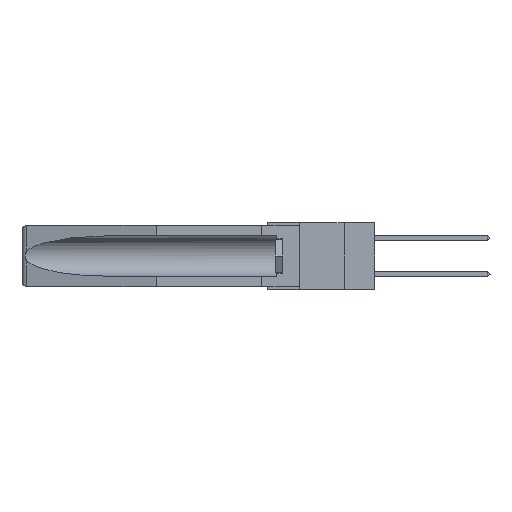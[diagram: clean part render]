
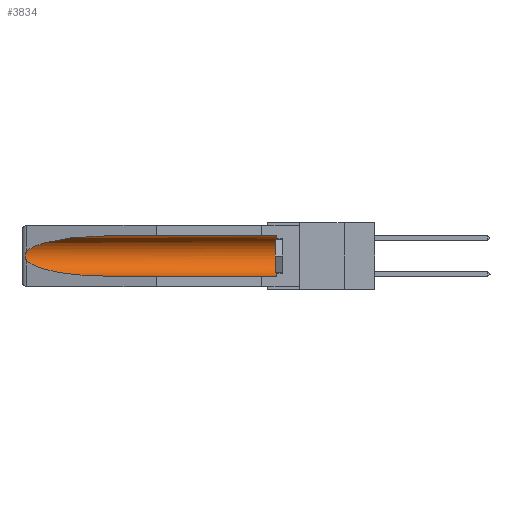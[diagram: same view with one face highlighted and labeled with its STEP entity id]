
A CAD part, left-side view. The second image highlights one B-rep face of the part: STEP entity #3834.
In plain terms, the highlighted cylindrical face has radius 2.857 mm (diameter 5.715 mm), a partial arc.
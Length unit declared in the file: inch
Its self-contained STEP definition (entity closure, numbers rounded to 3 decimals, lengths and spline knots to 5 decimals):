
#328 = ORIENTED_EDGE ( 'NONE', *, *, #12230, .T. ) ;
#489 = CARTESIAN_POINT ( 'NONE',  ( 0.155, 0.126, -0.284 ) ) ;
#1151 = AXIS2_PLACEMENT_3D ( 'NONE', #7534, #4968, #14448 ) ;
#1453 = EDGE_CURVE ( 'NONE', #27020, #3068, #8650, .T. ) ;
#1530 = CARTESIAN_POINT ( 'NONE',  ( 0.2673, 1.53269, -0.17917 ) ) ;
#1660 = CARTESIAN_POINT ( 'NONE',  ( 0.26537, 1.52718, -0.19328 ) ) ;
#2559 = CARTESIAN_POINT ( 'NONE',  ( 0.21114, 1.30732, -0.059 ) ) ;
#3068 = VERTEX_POINT ( 'NONE', #8744 ) ;
#3500 = VERTEX_POINT ( 'NONE', #16762 ) ;
#3834 = ADVANCED_FACE ( 'NONE', ( #11107 ), #24157, .F. ) ;
#3951 = CARTESIAN_POINT ( 'NONE',  ( 0.25451, 1.48313, -0.24835 ) ) ;
#4860 = CARTESIAN_POINT ( 'NONE',  ( 0.26537, 1.52718, -0.14972 ) ) ;
#4968 = DIRECTION ( 'NONE',  ( 0., -1., 0. ) ) ;
#6012 = CARTESIAN_POINT ( 'NONE',  ( 0.26537, 1.52718, -0.19328 ) ) ;
#6924 = ORIENTED_EDGE ( 'NONE', *, *, #9875, .T. ) ;
#7005 = ORIENTED_EDGE ( 'NONE', *, *, #20177, .T. ) ;
#7534 = CARTESIAN_POINT ( 'NONE',  ( 0.155, 0.126, -0.1715 ) ) ;
#8206 = CARTESIAN_POINT ( 'NONE',  ( 0.26537, 1.52718, -0.14972 ) ) ;
#8302 = CARTESIAN_POINT ( 'NONE',  ( 0.2675, 1.53308, -0.16763 ) ) ;
#8340 = CARTESIAN_POINT ( 'NONE',  ( 0.155, 1.07973, -0.284 ) ) ;
#8650 = CIRCLE ( 'NONE', #1151, 0.1125 ) ;
#8744 = CARTESIAN_POINT ( 'NONE',  ( 0.155, 0.126, -0.059 ) ) ;
#9875 = EDGE_CURVE ( 'NONE', #3500, #29275, #27918, .T. ) ;
#10318 = CARTESIAN_POINT ( 'NONE',  ( 0.21114, 1.30732, -0.284 ) ) ;
#10453 = LINE ( 'NONE', #14992, #12602 ) ;
#10569 = CARTESIAN_POINT ( 'NONE',  ( 0.2675, 1.53308, -0.17534 ) ) ;
#10689 = DIRECTION ( 'NONE',  ( 0., 1., 0. ) ) ;
#11107 = FACE_OUTER_BOUND ( 'NONE', #26128, .T. ) ;
#11844 = EDGE_CURVE ( 'NONE', #14674, #22599, #17428, .T. ) ;
#12136 = B_SPLINE_CURVE_WITH_KNOTS ( 'NONE', 3,
 ( #8206, #26309, #24010, #19602, #8302, #10569, #1530, #12877, #17172, #6012 ),
 .UNSPECIFIED., .F., .F.,
 ( 4, 2, 2, 2, 4 ),
 ( 0., 0.00029, 0.00058, 0.00087, 0.00117 ),
 .UNSPECIFIED. ) ;
#12230 = EDGE_CURVE ( 'NONE', #29275, #14674, #12136, .T. ) ;
#12359 = ORIENTED_EDGE ( 'NONE', *, *, #16674, .F. ) ;
#12436 = LINE ( 'NONE', #12764, #19887 ) ;
#12602 = VECTOR ( 'NONE', #10689, 39.37008 ) ;
#12764 = CARTESIAN_POINT ( 'NONE',  ( 0.155, -0.30754, -0.284 ) ) ;
#12877 = CARTESIAN_POINT ( 'NONE',  ( 0.26655, 1.53094, -0.18657 ) ) ;
#13582 = DIRECTION ( 'NONE',  ( 0., 1., 0. ) ) ;
#14448 = DIRECTION ( 'NONE',  ( 0., 0., 1. ) ) ;
#14674 = VERTEX_POINT ( 'NONE', #24189 ) ;
#14992 = CARTESIAN_POINT ( 'NONE',  ( 0.155, -0.30754, -0.059 ) ) ;
#15958 = CARTESIAN_POINT ( 'NONE',  ( 0.155, -0.30754, -0.1715 ) ) ;
#16184 = CARTESIAN_POINT ( 'NONE',  ( 0.155, 1.07973, -0.059 ) ) ;
#16664 = ORIENTED_EDGE ( 'NONE', *, *, #1453, .T. ) ;
#16674 = EDGE_CURVE ( 'NONE', #27020, #22599, #12436, .T. ) ;
#16762 = CARTESIAN_POINT ( 'NONE',  ( 0.155, 1.07973, -0.059 ) ) ;
#17172 = CARTESIAN_POINT ( 'NONE',  ( 0.26597, 1.5296, -0.19026 ) ) ;
#17428 =( BOUNDED_CURVE ( )  B_SPLINE_CURVE ( 3, ( #1660, #3951, #10318, #8340 ),
 .UNSPECIFIED., .F., .F. ) 
 B_SPLINE_CURVE_WITH_KNOTS ( ( 4, 4 ),
 ( 0.1948, 1.5708 ),
 .UNSPECIFIED. ) 
 CURVE ( )  GEOMETRIC_REPRESENTATION_ITEM ( )  RATIONAL_B_SPLINE_CURVE ( ( 1., 0.848, 0.848, 1. ) ) 
 REPRESENTATION_ITEM ( '' )  );
#18464 = CARTESIAN_POINT ( 'NONE',  ( 0.25451, 1.48313, -0.09465 ) ) ;
#19602 = CARTESIAN_POINT ( 'NONE',  ( 0.2673, 1.5327, -0.16383 ) ) ;
#19887 = VECTOR ( 'NONE', #21674, 39.37008 ) ;
#20177 = EDGE_CURVE ( 'NONE', #3068, #3500, #10453, .T. ) ;
#21674 = DIRECTION ( 'NONE',  ( 0., 1., 0. ) ) ;
#22599 = VERTEX_POINT ( 'NONE', #26052 ) ;
#24010 = CARTESIAN_POINT ( 'NONE',  ( 0.26654, 1.53092, -0.15636 ) ) ;
#24157 = CYLINDRICAL_SURFACE ( 'NONE', #28182, 0.1125 ) ;
#24189 = CARTESIAN_POINT ( 'NONE',  ( 0.26537, 1.52718, -0.19328 ) ) ;
#26052 = CARTESIAN_POINT ( 'NONE',  ( 0.155, 1.07973, -0.284 ) ) ;
#26128 = EDGE_LOOP ( 'NONE', ( #6924, #328, #27805, #12359, #16664, #7005 ) ) ;
#26309 = CARTESIAN_POINT ( 'NONE',  ( 0.26597, 1.52961, -0.15275 ) ) ;
#26440 = CARTESIAN_POINT ( 'NONE',  ( 0.26537, 1.52718, -0.14972 ) ) ;
#27020 = VERTEX_POINT ( 'NONE', #489 ) ;
#27805 = ORIENTED_EDGE ( 'NONE', *, *, #11844, .T. ) ;
#27843 = DIRECTION ( 'NONE',  ( 0., 0., 1. ) ) ;
#27918 =( BOUNDED_CURVE ( )  B_SPLINE_CURVE ( 3, ( #16184, #2559, #18464, #4860 ),
 .UNSPECIFIED., .F., .F. ) 
 B_SPLINE_CURVE_WITH_KNOTS ( ( 4, 4 ),
 ( 4.71239, 6.08839 ),
 .UNSPECIFIED. ) 
 CURVE ( )  GEOMETRIC_REPRESENTATION_ITEM ( )  RATIONAL_B_SPLINE_CURVE ( ( 1., 0.848, 0.848, 1. ) ) 
 REPRESENTATION_ITEM ( '' )  );
#28182 = AXIS2_PLACEMENT_3D ( 'NONE', #15958, #13582, #27843 ) ;
#29275 = VERTEX_POINT ( 'NONE', #26440 ) ;
